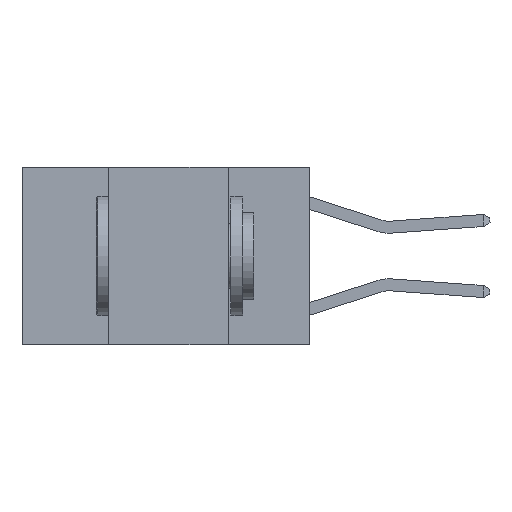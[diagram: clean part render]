
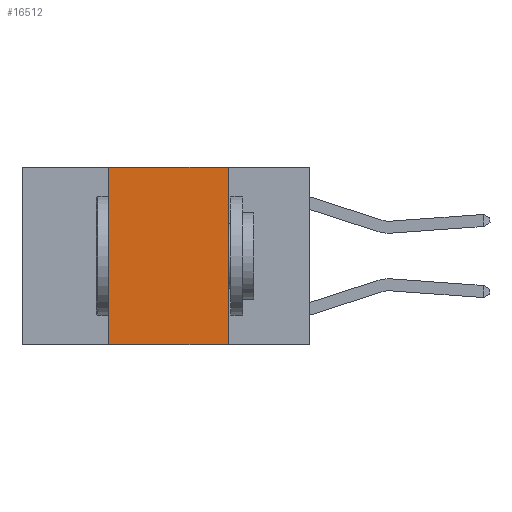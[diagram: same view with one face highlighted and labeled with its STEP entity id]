
A CAD part, left-side view. The second image highlights one B-rep face of the part: STEP entity #16512.
In plain terms, the highlighted planar face has unit normal (-1, 0, 0).
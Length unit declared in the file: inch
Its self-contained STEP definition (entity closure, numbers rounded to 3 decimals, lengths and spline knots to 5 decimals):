
#403 = AXIS2_PLACEMENT_3D ( 'NONE', #7949, #2111, #23091 ) ;
#1600 = CARTESIAN_POINT ( 'NONE',  ( 0., 0.42, 0. ) ) ;
#2111 = DIRECTION ( 'NONE',  ( 1., 0., 0. ) ) ;
#2608 = CARTESIAN_POINT ( 'NONE',  ( 0., 0.6, -0.37 ) ) ;
#2696 = VECTOR ( 'NONE', #13436, 39.37008 ) ;
#3240 = VERTEX_POINT ( 'NONE', #4263 ) ;
#4074 = EDGE_CURVE ( 'NONE', #11547, #3240, #23582, .T. ) ;
#4263 = CARTESIAN_POINT ( 'NONE',  ( 0., 0.17, -0.37 ) ) ;
#4573 = DIRECTION ( 'NONE',  ( 0., -1., 0. ) ) ;
#5302 = ORIENTED_EDGE ( 'NONE', *, *, #4074, .T. ) ;
#5961 = ORIENTED_EDGE ( 'NONE', *, *, #10858, .F. ) ;
#6576 = DIRECTION ( 'NONE',  ( 0., -1., 0. ) ) ;
#7842 = LINE ( 'NONE', #24662, #2696 ) ;
#7949 = CARTESIAN_POINT ( 'NONE',  ( 0., 0.6, 0. ) ) ;
#8508 = VECTOR ( 'NONE', #4573, 39.37008 ) ;
#9000 = FACE_OUTER_BOUND ( 'NONE', #9263, .T. ) ;
#9086 = VECTOR ( 'NONE', #15061, 39.37008 ) ;
#9263 = EDGE_LOOP ( 'NONE', ( #18964, #5961, #17507, #5302 ) ) ;
#9919 = PLANE ( 'NONE',  #403 ) ;
#10858 = EDGE_CURVE ( 'NONE', #24281, #11186, #24600, .T. ) ;
#11186 = VERTEX_POINT ( 'NONE', #20757 ) ;
#11547 = VERTEX_POINT ( 'NONE', #16077 ) ;
#13436 = DIRECTION ( 'NONE',  ( 0., 0., -1. ) ) ;
#14032 = VECTOR ( 'NONE', #6576, 39.37008 ) ;
#14219 = CARTESIAN_POINT ( 'NONE',  ( 0., 0.6, 0. ) ) ;
#14373 = EDGE_CURVE ( 'NONE', #11186, #3240, #7842, .T. ) ;
#15061 = DIRECTION ( 'NONE',  ( 0., 0., 1. ) ) ;
#16077 = CARTESIAN_POINT ( 'NONE',  ( 0., 0.42, -0.37 ) ) ;
#16512 = ADVANCED_FACE ( 'NONE', ( #9000 ), #9919, .F. ) ;
#17507 = ORIENTED_EDGE ( 'NONE', *, *, #21123, .F. ) ;
#18964 = ORIENTED_EDGE ( 'NONE', *, *, #14373, .F. ) ;
#19448 = CARTESIAN_POINT ( 'NONE',  ( 0., 0.42, 0. ) ) ;
#20757 = CARTESIAN_POINT ( 'NONE',  ( 0., 0.17, 0. ) ) ;
#21123 = EDGE_CURVE ( 'NONE', #11547, #24281, #24132, .T. ) ;
#23091 = DIRECTION ( 'NONE',  ( 0., 0., -1. ) ) ;
#23582 = LINE ( 'NONE', #2608, #8508 ) ;
#24132 = LINE ( 'NONE', #1600, #9086 ) ;
#24281 = VERTEX_POINT ( 'NONE', #19448 ) ;
#24600 = LINE ( 'NONE', #14219, #14032 ) ;
#24662 = CARTESIAN_POINT ( 'NONE',  ( 0., 0.17, 0. ) ) ;
